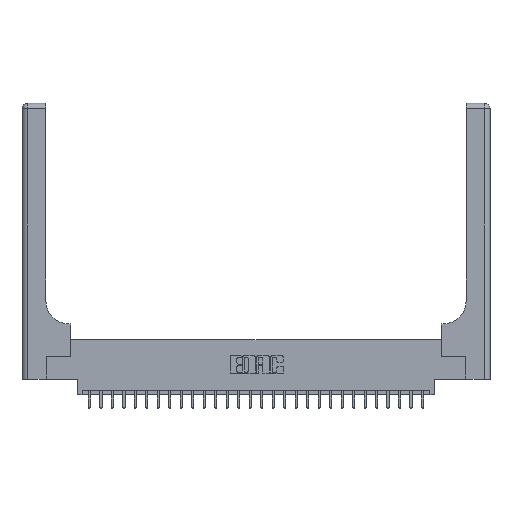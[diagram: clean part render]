
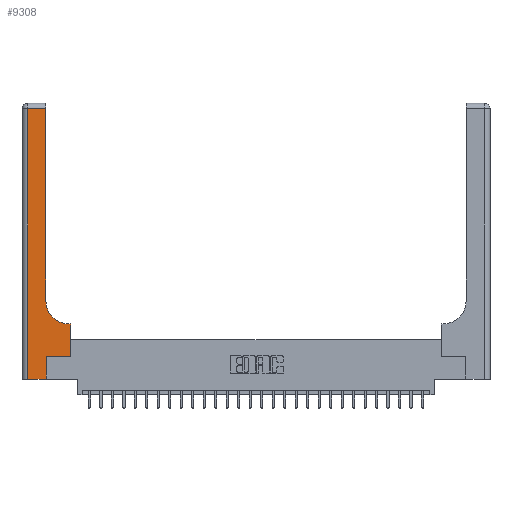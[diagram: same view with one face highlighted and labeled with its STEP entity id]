
A CAD part, top view. The second image highlights one B-rep face of the part: STEP entity #9308.
In plain terms, the highlighted planar face has unit normal (0, 0, 1).
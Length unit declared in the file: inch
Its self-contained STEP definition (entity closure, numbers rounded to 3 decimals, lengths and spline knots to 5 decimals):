
#184 = CARTESIAN_POINT ( 'NONE',  ( 0.528, 0.6, 0.37 ) ) ;
#253 = DIRECTION ( 'NONE',  ( 0., 1., 0. ) ) ;
#511 = VECTOR ( 'NONE', #253, 39.37008 ) ;
#716 = EDGE_CURVE ( 'NONE', #15982, #9975, #22747, .T. ) ;
#868 = PLANE ( 'NONE',  #2315 ) ;
#956 = EDGE_CURVE ( 'NONE', #11478, #22035, #2303, .T. ) ;
#1369 = CARTESIAN_POINT ( 'NONE',  ( 0.51, 0.6, 0.37 ) ) ;
#1792 = LINE ( 'NONE', #16373, #12427 ) ;
#1802 = DIRECTION ( 'NONE',  ( 1., 0., 0. ) ) ;
#1829 = ORIENTED_EDGE ( 'NONE', *, *, #17286, .T. ) ;
#1856 = ORIENTED_EDGE ( 'NONE', *, *, #19335, .T. ) ;
#1894 = VECTOR ( 'NONE', #25607, 39.37008 ) ;
#2303 = LINE ( 'NONE', #18957, #511 ) ;
#2304 = CARTESIAN_POINT ( 'NONE',  ( 0.528, 0.25, 0.37 ) ) ;
#2315 = AXIS2_PLACEMENT_3D ( 'NONE', #6847, #25386, #23331 ) ;
#2683 = EDGE_CURVE ( 'NONE', #9975, #23162, #26342, .T. ) ;
#3482 = ORIENTED_EDGE ( 'NONE', *, *, #956, .T. ) ;
#3611 = AXIS2_PLACEMENT_3D ( 'NONE', #20918, #8238, #20642 ) ;
#4550 = CARTESIAN_POINT ( 'NONE',  ( 0.06, 3., 0.37 ) ) ;
#4922 = ORIENTED_EDGE ( 'NONE', *, *, #716, .T. ) ;
#5137 = VECTOR ( 'NONE', #13932, 39.37008 ) ;
#5513 = DIRECTION ( 'NONE',  ( -1., 0., 0. ) ) ;
#5617 = CARTESIAN_POINT ( 'NONE',  ( 0.26, 0.6, 0.37 ) ) ;
#6460 = DIRECTION ( 'NONE',  ( 1., 0., 0. ) ) ;
#6763 = LINE ( 'NONE', #4550, #18424 ) ;
#6838 = LINE ( 'NONE', #15122, #21749 ) ;
#6847 = CARTESIAN_POINT ( 'NONE',  ( 0., 3., 0.37 ) ) ;
#6950 = EDGE_CURVE ( 'NONE', #23701, #15982, #1792, .T. ) ;
#7353 = CARTESIAN_POINT ( 'NONE',  ( 0.06, 2.94, 0.37 ) ) ;
#8238 = DIRECTION ( 'NONE',  ( 0., 0., -1. ) ) ;
#8705 = EDGE_CURVE ( 'NONE', #23162, #11478, #26692, .T. ) ;
#9226 = ORIENTED_EDGE ( 'NONE', *, *, #6950, .T. ) ;
#9232 = VERTEX_POINT ( 'NONE', #13697 ) ;
#9308 = ADVANCED_FACE ( 'NONE', ( #23660 ), #868, .F. ) ;
#9975 = VERTEX_POINT ( 'NONE', #184 ) ;
#10342 = CARTESIAN_POINT ( 'NONE',  ( 0.528, 0.25, 0.37 ) ) ;
#10981 = EDGE_CURVE ( 'NONE', #18166, #9232, #6763, .T. ) ;
#11006 = DIRECTION ( 'NONE',  ( 0., -1., 0. ) ) ;
#11478 = VERTEX_POINT ( 'NONE', #20258 ) ;
#12427 = VECTOR ( 'NONE', #6460, 39.37008 ) ;
#13102 = DIRECTION ( 'NONE',  ( 0., 1., 0. ) ) ;
#13160 = ORIENTED_EDGE ( 'NONE', *, *, #8705, .T. ) ;
#13697 = CARTESIAN_POINT ( 'NONE',  ( 0.06, 0., 0.37 ) ) ;
#13932 = DIRECTION ( 'NONE',  ( -1., 0., 0. ) ) ;
#14699 = CARTESIAN_POINT ( 'NONE',  ( 0.26, 2.94, 0.37 ) ) ;
#14778 = EDGE_LOOP ( 'NONE', ( #3482, #25020, #14966, #1829, #1856, #9226, #4922, #15184, #13160 ) ) ;
#14966 = ORIENTED_EDGE ( 'NONE', *, *, #10981, .T. ) ;
#15122 = CARTESIAN_POINT ( 'NONE',  ( 0.265, 0., 0.37 ) ) ;
#15184 = ORIENTED_EDGE ( 'NONE', *, *, #2683, .T. ) ;
#15390 = EDGE_CURVE ( 'NONE', #22035, #18166, #20357, .T. ) ;
#15982 = VERTEX_POINT ( 'NONE', #2304 ) ;
#16373 = CARTESIAN_POINT ( 'NONE',  ( 0.265, 0.25, 0.37 ) ) ;
#17286 = EDGE_CURVE ( 'NONE', #9232, #25910, #24463, .T. ) ;
#18166 = VERTEX_POINT ( 'NONE', #7353 ) ;
#18275 = CARTESIAN_POINT ( 'NONE',  ( 0.265, 0.25, 0.37 ) ) ;
#18332 = CARTESIAN_POINT ( 'NONE',  ( 0., 2.94, 0.37 ) ) ;
#18424 = VECTOR ( 'NONE', #11006, 39.37008 ) ;
#18957 = CARTESIAN_POINT ( 'NONE',  ( 0.26, 3., 0.37 ) ) ;
#19335 = EDGE_CURVE ( 'NONE', #25910, #23701, #6838, .T. ) ;
#20258 = CARTESIAN_POINT ( 'NONE',  ( 0.26, 0.85, 0.37 ) ) ;
#20357 = LINE ( 'NONE', #18332, #24112 ) ;
#20642 = DIRECTION ( 'NONE',  ( 1., 0., 0. ) ) ;
#20918 = CARTESIAN_POINT ( 'NONE',  ( 0.51, 0.85, 0.37 ) ) ;
#21749 = VECTOR ( 'NONE', #13102, 39.37008 ) ;
#22035 = VERTEX_POINT ( 'NONE', #14699 ) ;
#22747 = LINE ( 'NONE', #10342, #1894 ) ;
#23162 = VERTEX_POINT ( 'NONE', #1369 ) ;
#23331 = DIRECTION ( 'NONE',  ( -1., 0., 0. ) ) ;
#23660 = FACE_OUTER_BOUND ( 'NONE', #14778, .T. ) ;
#23701 = VERTEX_POINT ( 'NONE', #18275 ) ;
#24112 = VECTOR ( 'NONE', #5513, 39.37008 ) ;
#24338 = VECTOR ( 'NONE', #1802, 39.37008 ) ;
#24463 = LINE ( 'NONE', #24729, #24338 ) ;
#24616 = CARTESIAN_POINT ( 'NONE',  ( 0.265, 0., 0.37 ) ) ;
#24729 = CARTESIAN_POINT ( 'NONE',  ( 0., 0., 0.37 ) ) ;
#25020 = ORIENTED_EDGE ( 'NONE', *, *, #15390, .T. ) ;
#25386 = DIRECTION ( 'NONE',  ( 0., 0., -1. ) ) ;
#25607 = DIRECTION ( 'NONE',  ( 0., 1., 0. ) ) ;
#25910 = VERTEX_POINT ( 'NONE', #24616 ) ;
#26342 = LINE ( 'NONE', #5617, #5137 ) ;
#26692 = CIRCLE ( 'NONE', #3611, 0.25 ) ;
